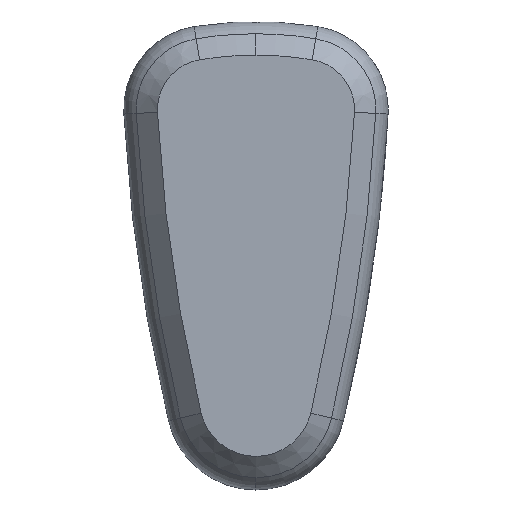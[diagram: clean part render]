
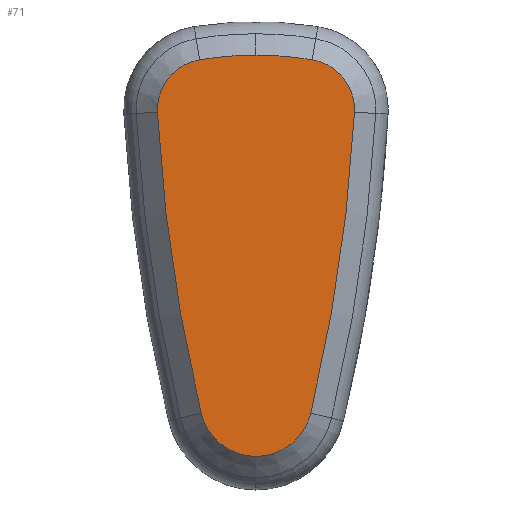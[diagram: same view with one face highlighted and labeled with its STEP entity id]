
A CAD part, front view. The second image highlights one B-rep face of the part: STEP entity #71.
In plain terms, the highlighted planar face has unit normal (0, -1, 0).
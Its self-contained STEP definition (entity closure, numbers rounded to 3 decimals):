
#1 = DIRECTION ( 'NONE',  ( 0., -1., 0. ) ) ;
#7 = CARTESIAN_POINT ( 'NONE',  ( 1.429, 0., 11.307 ) ) ;
#8 = VERTEX_POINT ( 'NONE', #547 ) ;
#17 = DIRECTION ( 'NONE',  ( 0., 0., -1. ) ) ;
#21 = DIRECTION ( 'NONE',  ( 0., -1., 0. ) ) ;
#32 = CARTESIAN_POINT ( 'NONE',  ( -47.081, 0., 13.925 ) ) ;
#43 = DIRECTION ( 'NONE',  ( 0., 0., -1. ) ) ;
#52 = DIRECTION ( 'NONE',  ( 0., -1., 0. ) ) ;
#55 = CARTESIAN_POINT ( 'NONE',  ( 0., 0., 2.675 ) ) ;
#64 = ORIENTED_EDGE ( 'NONE', *, *, #816, .T. ) ;
#69 = DIRECTION ( 'NONE',  ( 0., 0., -1. ) ) ;
#71 = ADVANCED_FACE ( 'NONE', ( #786 ), #261, .T. ) ;
#72 = DIRECTION ( 'NONE',  ( 0., -1., 0. ) ) ;
#81 = EDGE_CURVE ( 'NONE', #661, #94, #759, .T. ) ;
#84 = CARTESIAN_POINT ( 'NONE',  ( 47.081, 0., 13.925 ) ) ;
#94 = VERTEX_POINT ( 'NONE', #148 ) ;
#95 = EDGE_CURVE ( 'NONE', #763, #8, #745, .T. ) ;
#98 = EDGE_CURVE ( 'NONE', #8, #877, #762, .T. ) ;
#101 = DIRECTION ( 'NONE',  ( 0., 0., -1. ) ) ;
#103 = DIRECTION ( 'NONE',  ( 0., -1., 0. ) ) ;
#105 = CARTESIAN_POINT ( 'NONE',  ( -1.429, 0., 11.307 ) ) ;
#107 = EDGE_CURVE ( 'NONE', #877, #823, #747, .T. ) ;
#110 = EDGE_CURVE ( 'NONE', #823, #193, #738, .T. ) ;
#111 = EDGE_CURVE ( 'NONE', #193, #661, #737, .T. ) ;
#148 = CARTESIAN_POINT ( 'NONE',  ( 0., 0., 12.925 ) ) ;
#151 = DIRECTION ( 'NONE',  ( 0., -1., 0. ) ) ;
#178 = DIRECTION ( 'NONE',  ( 0., 0., -1. ) ) ;
#180 = CARTESIAN_POINT ( 'NONE',  ( 2.927, 0., 11.226 ) ) ;
#182 = DIRECTION ( 'NONE',  ( 0., -1., 0. ) ) ;
#187 = CARTESIAN_POINT ( 'NONE',  ( 0., 0., 2.675 ) ) ;
#193 = VERTEX_POINT ( 'NONE', #180 ) ;
#205 = EDGE_LOOP ( 'NONE', ( #921, #64, #413, #412, #890, #207, #347 ) ) ;
#206 = CARTESIAN_POINT ( 'NONE',  ( 1.674, 0., 12.787 ) ) ;
#207 = ORIENTED_EDGE ( 'NONE', *, *, #110, .T. ) ;
#255 = DIRECTION ( 'NONE',  ( 0., 0., -1. ) ) ;
#259 = DIRECTION ( 'NONE',  ( 0., -1., 0. ) ) ;
#261 = PLANE ( 'NONE',  #327 ) ;
#287 = CARTESIAN_POINT ( 'NONE',  ( 4., 0., 0. ) ) ;
#327 = AXIS2_PLACEMENT_3D ( 'NONE', #287, #259, #255 ) ;
#347 = ORIENTED_EDGE ( 'NONE', *, *, #111, .T. ) ;
#412 = ORIENTED_EDGE ( 'NONE', *, *, #98, .T. ) ;
#413 = ORIENTED_EDGE ( 'NONE', *, *, #95, .T. ) ;
#415 = CIRCLE ( 'NONE', #846, 10.25 ) ;
#448 = AXIS2_PLACEMENT_3D ( 'NONE', #187, #182, #178 ) ;
#547 = CARTESIAN_POINT ( 'NONE',  ( -2.927, 0., 11.226 ) ) ;
#576 = DIRECTION ( 'NONE',  ( 0., 0., -1. ) ) ;
#616 = CARTESIAN_POINT ( 'NONE',  ( -1.674, 0., 12.787 ) ) ;
#626 = CARTESIAN_POINT ( 'NONE',  ( 0., 0., 2.675 ) ) ;
#654 = AXIS2_PLACEMENT_3D ( 'NONE', #105, #103, #101 ) ;
#661 = VERTEX_POINT ( 'NONE', #206 ) ;
#701 = CARTESIAN_POINT ( 'NONE',  ( 1.629, 0., 2.285 ) ) ;
#704 = DIRECTION ( 'NONE',  ( 0., 0., -1. ) ) ;
#705 = AXIS2_PLACEMENT_3D ( 'NONE', #84, #72, #69 ) ;
#708 = CARTESIAN_POINT ( 'NONE',  ( -1.629, 0., 2.285 ) ) ;
#737 = CIRCLE ( 'NONE', #850, 1.5 ) ;
#738 = CIRCLE ( 'NONE', #801, 50.081 ) ;
#745 = CIRCLE ( 'NONE', #654, 1.5 ) ;
#746 = AXIS2_PLACEMENT_3D ( 'NONE', #55, #52, #43 ) ;
#747 = CIRCLE ( 'NONE', #746, 1.675 ) ;
#759 = CIRCLE ( 'NONE', #448, 10.25 ) ;
#762 = CIRCLE ( 'NONE', #705, 50.081 ) ;
#763 = VERTEX_POINT ( 'NONE', #616 ) ;
#786 = FACE_OUTER_BOUND ( 'NONE', #205, .T. ) ;
#801 = AXIS2_PLACEMENT_3D ( 'NONE', #32, #21, #17 ) ;
#816 = EDGE_CURVE ( 'NONE', #94, #763, #415, .T. ) ;
#823 = VERTEX_POINT ( 'NONE', #701 ) ;
#846 = AXIS2_PLACEMENT_3D ( 'NONE', #626, #151, #704 ) ;
#850 = AXIS2_PLACEMENT_3D ( 'NONE', #7, #1, #576 ) ;
#877 = VERTEX_POINT ( 'NONE', #708 ) ;
#890 = ORIENTED_EDGE ( 'NONE', *, *, #107, .T. ) ;
#921 = ORIENTED_EDGE ( 'NONE', *, *, #81, .T. ) ;
